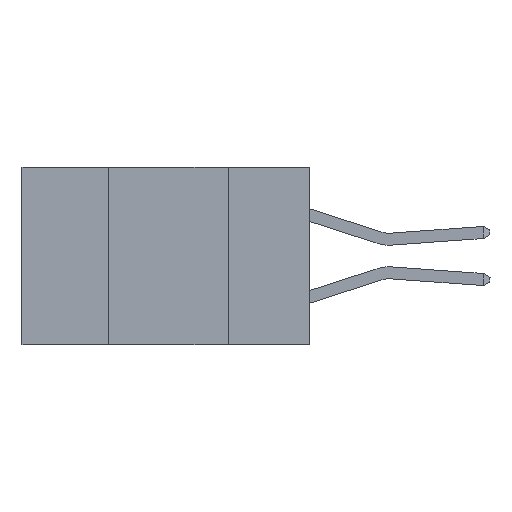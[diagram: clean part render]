
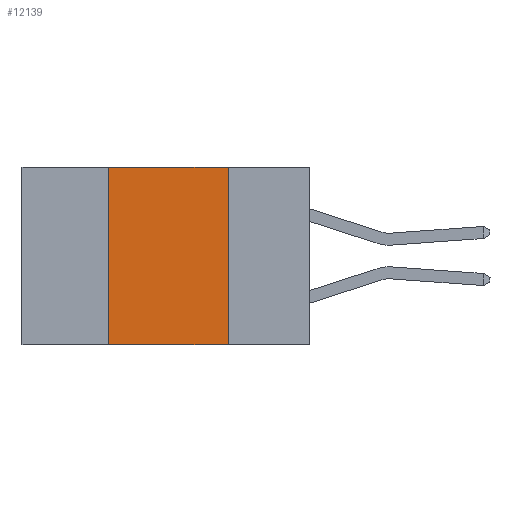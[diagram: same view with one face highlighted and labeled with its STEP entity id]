
A CAD part, left-side view. The second image highlights one B-rep face of the part: STEP entity #12139.
In plain terms, the highlighted planar face has unit normal (-1, 0, 0).
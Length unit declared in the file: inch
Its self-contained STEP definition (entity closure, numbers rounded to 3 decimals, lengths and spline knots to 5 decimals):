
#117 = DIRECTION ( 'NONE',  ( 0., -1., 0. ) ) ;
#138 = CARTESIAN_POINT ( 'NONE',  ( 0., 0.6, -0.37 ) ) ;
#423 = ORIENTED_EDGE ( 'NONE', *, *, #8963, .T. ) ;
#529 = AXIS2_PLACEMENT_3D ( 'NONE', #5831, #7725, #20839 ) ;
#1082 = CARTESIAN_POINT ( 'NONE',  ( 0., 0.42, -0.37 ) ) ;
#3057 = EDGE_CURVE ( 'NONE', #5282, #14706, #21470, .T. ) ;
#3534 = FACE_OUTER_BOUND ( 'NONE', #16126, .T. ) ;
#3647 = DIRECTION ( 'NONE',  ( 0., 0., -1. ) ) ;
#4015 = EDGE_CURVE ( 'NONE', #9385, #17004, #15828, .T. ) ;
#4659 = ORIENTED_EDGE ( 'NONE', *, *, #23178, .F. ) ;
#5282 = VERTEX_POINT ( 'NONE', #20451 ) ;
#5831 = CARTESIAN_POINT ( 'NONE',  ( 0., 0.6, 0. ) ) ;
#5925 = DIRECTION ( 'NONE',  ( 0., -1., 0. ) ) ;
#7725 = DIRECTION ( 'NONE',  ( 1., 0., 0. ) ) ;
#8963 = EDGE_CURVE ( 'NONE', #5282, #17004, #13414, .T. ) ;
#9385 = VERTEX_POINT ( 'NONE', #9608 ) ;
#9608 = CARTESIAN_POINT ( 'NONE',  ( 0., 0.17, 0. ) ) ;
#11864 = ORIENTED_EDGE ( 'NONE', *, *, #4015, .F. ) ;
#12139 = ADVANCED_FACE ( 'NONE', ( #3534 ), #13344, .F. ) ;
#12178 = VECTOR ( 'NONE', #18043, 39.37008 ) ;
#13344 = PLANE ( 'NONE',  #529 ) ;
#13414 = LINE ( 'NONE', #138, #16558 ) ;
#13515 = CARTESIAN_POINT ( 'NONE',  ( 0., 0.42, 0. ) ) ;
#14706 = VERTEX_POINT ( 'NONE', #13515 ) ;
#14725 = LINE ( 'NONE', #18936, #19112 ) ;
#15828 = LINE ( 'NONE', #16756, #19671 ) ;
#16126 = EDGE_LOOP ( 'NONE', ( #11864, #4659, #18730, #423 ) ) ;
#16558 = VECTOR ( 'NONE', #5925, 39.37008 ) ;
#16756 = CARTESIAN_POINT ( 'NONE',  ( 0., 0.17, -0.37 ) ) ;
#17004 = VERTEX_POINT ( 'NONE', #19791 ) ;
#18043 = DIRECTION ( 'NONE',  ( 0., 0., 1. ) ) ;
#18730 = ORIENTED_EDGE ( 'NONE', *, *, #3057, .F. ) ;
#18936 = CARTESIAN_POINT ( 'NONE',  ( 0., 0.6, 0. ) ) ;
#19112 = VECTOR ( 'NONE', #117, 39.37008 ) ;
#19671 = VECTOR ( 'NONE', #3647, 39.37008 ) ;
#19791 = CARTESIAN_POINT ( 'NONE',  ( 0., 0.17, -0.37 ) ) ;
#20451 = CARTESIAN_POINT ( 'NONE',  ( 0., 0.42, -0.37 ) ) ;
#20839 = DIRECTION ( 'NONE',  ( 0., 0., -1. ) ) ;
#21470 = LINE ( 'NONE', #1082, #12178 ) ;
#23178 = EDGE_CURVE ( 'NONE', #14706, #9385, #14725, .T. ) ;
